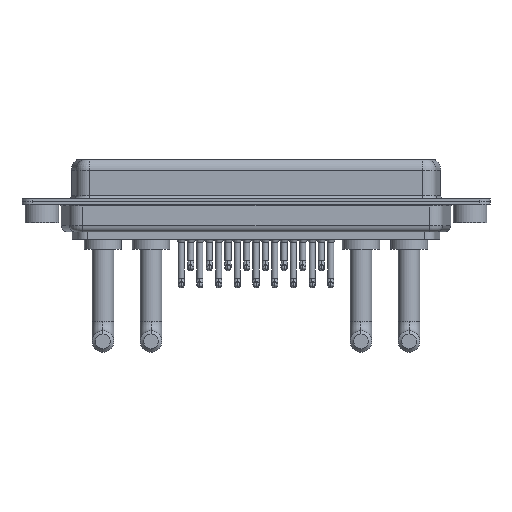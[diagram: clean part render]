
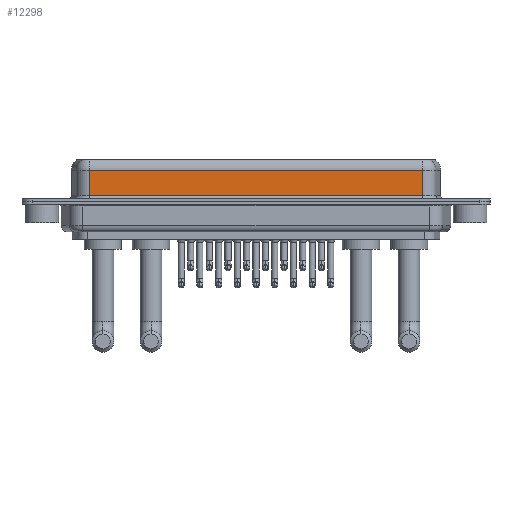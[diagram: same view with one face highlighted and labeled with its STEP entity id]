
A CAD part, front view. The second image highlights one B-rep face of the part: STEP entity #12298.
In plain terms, the highlighted planar face has unit normal (0, -1, 0).
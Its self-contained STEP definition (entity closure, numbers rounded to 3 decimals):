
#1007 = CARTESIAN_POINT ( 'NONE',  ( 7.038, -3.95, 6.4 ) ) ;
#1179 = EDGE_CURVE ( 'NONE', #9242, #4081, #11676, .T. ) ;
#1765 = CARTESIAN_POINT ( 'NONE',  ( 7.038, -3.95, 0.9 ) ) ;
#2008 = CARTESIAN_POINT ( 'NONE',  ( 56.462, -3.95, 0.9 ) ) ;
#2881 = CARTESIAN_POINT ( 'NONE',  ( 56.462, -3.95, 0.9 ) ) ;
#4081 = VERTEX_POINT ( 'NONE', #2008 ) ;
#4353 = LINE ( 'NONE', #1007, #10696 ) ;
#4512 = CARTESIAN_POINT ( 'NONE',  ( 56.462, -3.95, 4.65 ) ) ;
#4956 = DIRECTION ( 'NONE',  ( 0., 1., 0. ) ) ;
#5269 = ORIENTED_EDGE ( 'NONE', *, *, #8672, .F. ) ;
#5897 = CARTESIAN_POINT ( 'NONE',  ( 56.462, -3.95, 6.4 ) ) ;
#6090 = EDGE_CURVE ( 'NONE', #7805, #9242, #4353, .T. ) ;
#6448 = DIRECTION ( 'NONE',  ( 1., 0., 0. ) ) ;
#6506 = DIRECTION ( 'NONE',  ( 0., 0., 1. ) ) ;
#6834 = FACE_OUTER_BOUND ( 'NONE', #12632, .T. ) ;
#7738 = LINE ( 'NONE', #4512, #20386 ) ;
#7805 = VERTEX_POINT ( 'NONE', #14465 ) ;
#7902 = VERTEX_POINT ( 'NONE', #8114 ) ;
#8114 = CARTESIAN_POINT ( 'NONE',  ( 56.462, -3.95, 4.65 ) ) ;
#8173 = PLANE ( 'NONE',  #21844 ) ;
#8672 = EDGE_CURVE ( 'NONE', #7902, #4081, #13007, .T. ) ;
#9128 = VECTOR ( 'NONE', #6448, 1000. ) ;
#9242 = VERTEX_POINT ( 'NONE', #1765 ) ;
#10696 = VECTOR ( 'NONE', #19258, 1000. ) ;
#11094 = ORIENTED_EDGE ( 'NONE', *, *, #1179, .T. ) ;
#11293 = DIRECTION ( 'NONE',  ( -1., 0., 0. ) ) ;
#11337 = DIRECTION ( 'NONE',  ( 0., 0., -1. ) ) ;
#11439 = EDGE_CURVE ( 'NONE', #7902, #7805, #7738, .T. ) ;
#11676 = LINE ( 'NONE', #2881, #9128 ) ;
#12298 = ADVANCED_FACE ( 'NONE', ( #6834 ), #8173, .F. ) ;
#12328 = ORIENTED_EDGE ( 'NONE', *, *, #11439, .T. ) ;
#12632 = EDGE_LOOP ( 'NONE', ( #5269, #12328, #15339, #11094 ) ) ;
#13007 = LINE ( 'NONE', #5897, #15648 ) ;
#14465 = CARTESIAN_POINT ( 'NONE',  ( 7.038, -3.95, 4.65 ) ) ;
#14968 = CARTESIAN_POINT ( 'NONE',  ( 56.462, -3.95, 6.4 ) ) ;
#15339 = ORIENTED_EDGE ( 'NONE', *, *, #6090, .T. ) ;
#15648 = VECTOR ( 'NONE', #11337, 1000. ) ;
#19258 = DIRECTION ( 'NONE',  ( 0., 0., -1. ) ) ;
#20386 = VECTOR ( 'NONE', #11293, 1000. ) ;
#21844 = AXIS2_PLACEMENT_3D ( 'NONE', #14968, #4956, #6506 ) ;
